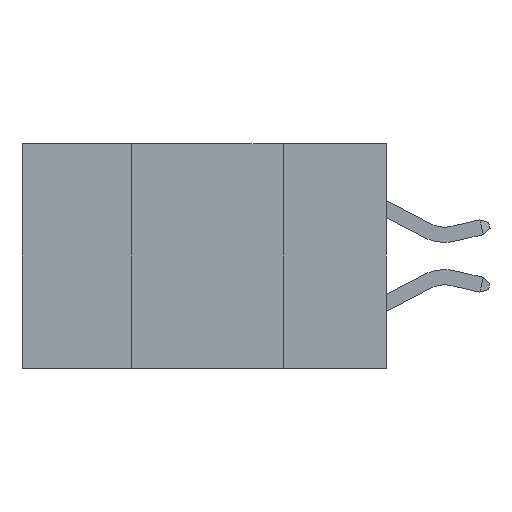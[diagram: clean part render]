
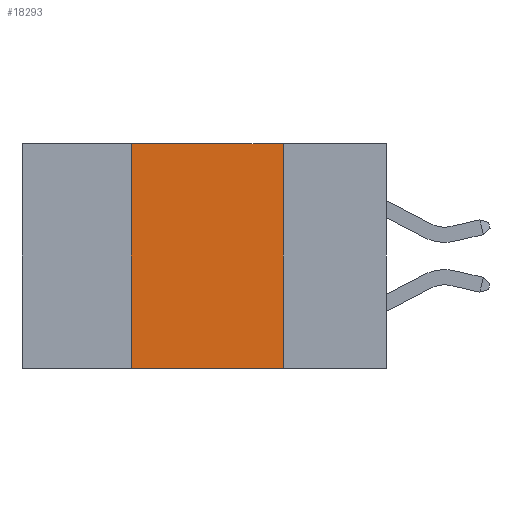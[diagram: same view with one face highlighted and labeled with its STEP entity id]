
A CAD part, left-side view. The second image highlights one B-rep face of the part: STEP entity #18293.
In plain terms, the highlighted planar face has unit normal (-1, 0, 0).
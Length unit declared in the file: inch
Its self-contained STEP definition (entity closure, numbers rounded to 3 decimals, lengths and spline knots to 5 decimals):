
#526 = VERTEX_POINT ( 'NONE', #11212 ) ;
#1083 = CARTESIAN_POINT ( 'NONE',  ( 0., 0.17, 0. ) ) ;
#1979 = CARTESIAN_POINT ( 'NONE',  ( 0., 0.6, -0.37 ) ) ;
#2063 = ORIENTED_EDGE ( 'NONE', *, *, #10049, .F. ) ;
#3184 = PLANE ( 'NONE',  #23103 ) ;
#3282 = DIRECTION ( 'NONE',  ( 0., 0., 1. ) ) ;
#3329 = ORIENTED_EDGE ( 'NONE', *, *, #12512, .F. ) ;
#4635 = EDGE_CURVE ( 'NONE', #10697, #25611, #24304, .T. ) ;
#5223 = LINE ( 'NONE', #17245, #21100 ) ;
#5922 = VERTEX_POINT ( 'NONE', #1083 ) ;
#5976 = EDGE_CURVE ( 'NONE', #10697, #526, #5223, .T. ) ;
#7216 = DIRECTION ( 'NONE',  ( 1., 0., 0. ) ) ;
#10049 = EDGE_CURVE ( 'NONE', #5922, #25611, #10657, .T. ) ;
#10657 = LINE ( 'NONE', #11576, #15322 ) ;
#10697 = VERTEX_POINT ( 'NONE', #17534 ) ;
#11212 = CARTESIAN_POINT ( 'NONE',  ( 0., 0.42, 0. ) ) ;
#11576 = CARTESIAN_POINT ( 'NONE',  ( 0., 0.17, 0. ) ) ;
#12512 = EDGE_CURVE ( 'NONE', #526, #5922, #24786, .T. ) ;
#13045 = VECTOR ( 'NONE', #20781, 39.37008 ) ;
#13414 = FACE_OUTER_BOUND ( 'NONE', #15774, .T. ) ;
#13980 = ORIENTED_EDGE ( 'NONE', *, *, #5976, .F. ) ;
#14832 = CARTESIAN_POINT ( 'NONE',  ( 0., 0.6, 0. ) ) ;
#15322 = VECTOR ( 'NONE', #25382, 39.37008 ) ;
#15774 = EDGE_LOOP ( 'NONE', ( #2063, #3329, #13980, #25687 ) ) ;
#17245 = CARTESIAN_POINT ( 'NONE',  ( 0., 0.42, 0. ) ) ;
#17534 = CARTESIAN_POINT ( 'NONE',  ( 0., 0.42, -0.37 ) ) ;
#17960 = DIRECTION ( 'NONE',  ( 0., -1., 0. ) ) ;
#18293 = ADVANCED_FACE ( 'NONE', ( #13414 ), #3184, .F. ) ;
#19082 = VECTOR ( 'NONE', #17960, 39.37008 ) ;
#19134 = CARTESIAN_POINT ( 'NONE',  ( 0., 0.6, 0. ) ) ;
#20781 = DIRECTION ( 'NONE',  ( 0., -1., 0. ) ) ;
#21056 = CARTESIAN_POINT ( 'NONE',  ( 0., 0.17, -0.37 ) ) ;
#21100 = VECTOR ( 'NONE', #3282, 39.37008 ) ;
#21102 = DIRECTION ( 'NONE',  ( 0., 0., -1. ) ) ;
#23103 = AXIS2_PLACEMENT_3D ( 'NONE', #19134, #7216, #21102 ) ;
#24304 = LINE ( 'NONE', #1979, #19082 ) ;
#24786 = LINE ( 'NONE', #14832, #13045 ) ;
#25382 = DIRECTION ( 'NONE',  ( 0., 0., -1. ) ) ;
#25611 = VERTEX_POINT ( 'NONE', #21056 ) ;
#25687 = ORIENTED_EDGE ( 'NONE', *, *, #4635, .T. ) ;
